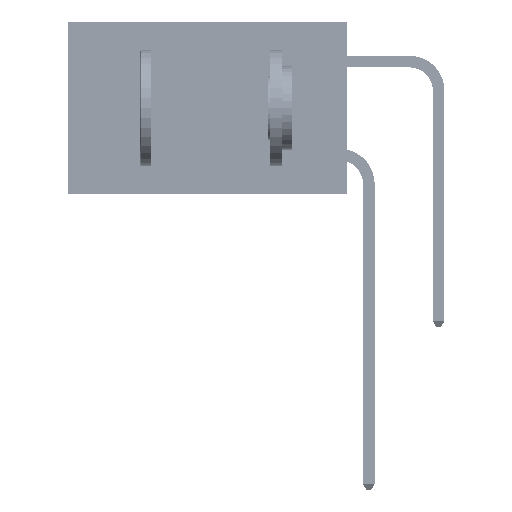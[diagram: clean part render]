
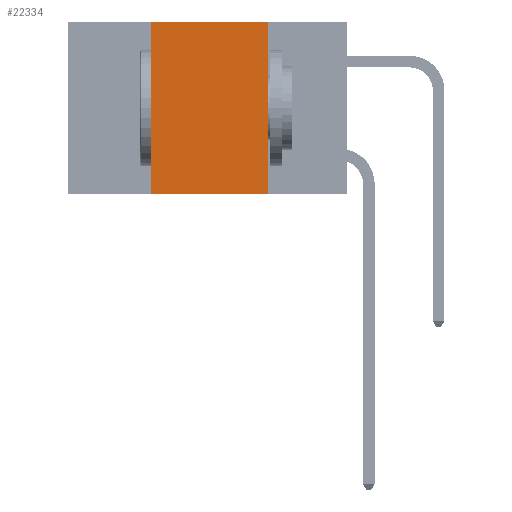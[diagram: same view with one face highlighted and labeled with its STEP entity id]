
A CAD part, left-side view. The second image highlights one B-rep face of the part: STEP entity #22334.
In plain terms, the highlighted planar face has unit normal (-1, 0, 0).
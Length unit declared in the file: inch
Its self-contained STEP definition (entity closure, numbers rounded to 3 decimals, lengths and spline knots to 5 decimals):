
#556 = CARTESIAN_POINT ( 'NONE',  ( 0., 0.6, 0. ) ) ;
#5285 = VERTEX_POINT ( 'NONE', #16798 ) ;
#5575 = VERTEX_POINT ( 'NONE', #27170 ) ;
#6744 = VECTOR ( 'NONE', #13986, 39.37008 ) ;
#10616 = EDGE_CURVE ( 'NONE', #53990, #44846, #19800, .T. ) ;
#13365 = DIRECTION ( 'NONE',  ( 0., 0., -1. ) ) ;
#13986 = DIRECTION ( 'NONE',  ( 0., -1., 0. ) ) ;
#14910 = ORIENTED_EDGE ( 'NONE', *, *, #21741, .T. ) ;
#15113 = VECTOR ( 'NONE', #53935, 39.37008 ) ;
#16798 = CARTESIAN_POINT ( 'NONE',  ( 0., 0.42, -0.37 ) ) ;
#17024 = CARTESIAN_POINT ( 'NONE',  ( 0., 0.17, 0. ) ) ;
#18024 = CARTESIAN_POINT ( 'NONE',  ( 0., 0.42, 0. ) ) ;
#19722 = LINE ( 'NONE', #28413, #15113 ) ;
#19800 = LINE ( 'NONE', #30575, #29775 ) ;
#21277 = EDGE_CURVE ( 'NONE', #5285, #53990, #24310, .T. ) ;
#21741 = EDGE_CURVE ( 'NONE', #5285, #5575, #28007, .T. ) ;
#22334 = ADVANCED_FACE ( 'NONE', ( #24643 ), #34685, .F. ) ;
#24310 = LINE ( 'NONE', #49792, #29656 ) ;
#24643 = FACE_OUTER_BOUND ( 'NONE', #41492, .T. ) ;
#25086 = EDGE_CURVE ( 'NONE', #44846, #5575, #19722, .T. ) ;
#25918 = DIRECTION ( 'NONE',  ( 0., -1., 0. ) ) ;
#27170 = CARTESIAN_POINT ( 'NONE',  ( 0., 0.17, -0.37 ) ) ;
#28007 = LINE ( 'NONE', #39381, #6744 ) ;
#28331 = DIRECTION ( 'NONE',  ( 0., 0., 1. ) ) ;
#28413 = CARTESIAN_POINT ( 'NONE',  ( 0., 0.17, 0. ) ) ;
#29656 = VECTOR ( 'NONE', #28331, 39.37008 ) ;
#29775 = VECTOR ( 'NONE', #25918, 39.37008 ) ;
#30575 = CARTESIAN_POINT ( 'NONE',  ( 0., 0.6, 0. ) ) ;
#31958 = ORIENTED_EDGE ( 'NONE', *, *, #21277, .F. ) ;
#33970 = ORIENTED_EDGE ( 'NONE', *, *, #10616, .F. ) ;
#34685 = PLANE ( 'NONE',  #44518 ) ;
#39381 = CARTESIAN_POINT ( 'NONE',  ( 0., 0.6, -0.37 ) ) ;
#41492 = EDGE_LOOP ( 'NONE', ( #51402, #33970, #31958, #14910 ) ) ;
#43600 = DIRECTION ( 'NONE',  ( 1., 0., 0. ) ) ;
#44518 = AXIS2_PLACEMENT_3D ( 'NONE', #556, #43600, #13365 ) ;
#44846 = VERTEX_POINT ( 'NONE', #17024 ) ;
#49792 = CARTESIAN_POINT ( 'NONE',  ( 0., 0.42, 0. ) ) ;
#51402 = ORIENTED_EDGE ( 'NONE', *, *, #25086, .F. ) ;
#53935 = DIRECTION ( 'NONE',  ( 0., 0., -1. ) ) ;
#53990 = VERTEX_POINT ( 'NONE', #18024 ) ;
